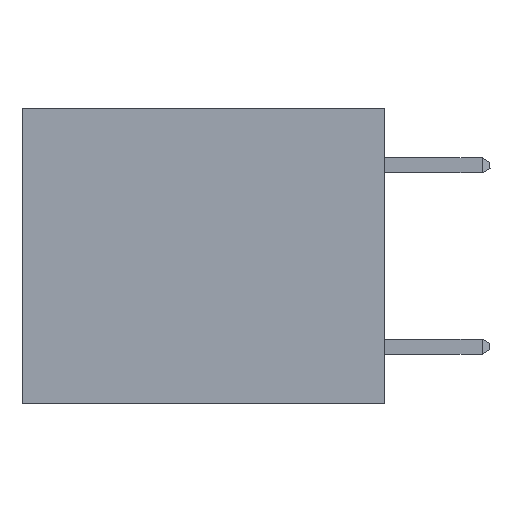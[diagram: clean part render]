
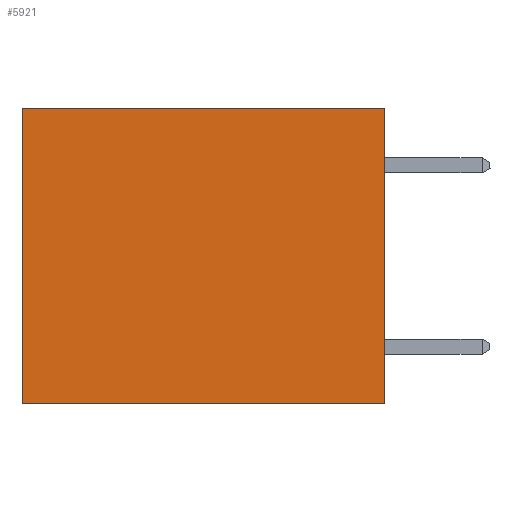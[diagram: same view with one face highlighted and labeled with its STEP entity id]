
A CAD part, left-side view. The second image highlights one B-rep face of the part: STEP entity #5921.
In plain terms, the highlighted planar face has unit normal (-1, 0, 0).
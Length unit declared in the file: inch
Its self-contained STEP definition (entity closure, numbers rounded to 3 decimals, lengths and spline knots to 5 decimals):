
#1148 = PLANE ( 'NONE',  #30560 ) ;
#2195 = ORIENTED_EDGE ( 'NONE', *, *, #9939, .F. ) ;
#3368 = CARTESIAN_POINT ( 'NONE',  ( 0.3165, 0., -0.49 ) ) ;
#4764 = DIRECTION ( 'NONE',  ( 0., 0., -1. ) ) ;
#5921 = ADVANCED_FACE ( 'NONE', ( #30733 ), #1148, .F. ) ;
#6543 = LINE ( 'NONE', #24455, #24176 ) ;
#6935 = VECTOR ( 'NONE', #18774, 39.37008 ) ;
#8947 = CARTESIAN_POINT ( 'NONE',  ( 0.3165, 0., -0.49 ) ) ;
#9203 = CARTESIAN_POINT ( 'NONE',  ( 0.3165, 0., 0. ) ) ;
#9793 = LINE ( 'NONE', #22160, #30605 ) ;
#9939 = EDGE_CURVE ( 'NONE', #31542, #16317, #9793, .T. ) ;
#10577 = ORIENTED_EDGE ( 'NONE', *, *, #11496, .F. ) ;
#10860 = VERTEX_POINT ( 'NONE', #31512 ) ;
#11496 = EDGE_CURVE ( 'NONE', #16317, #10860, #31246, .T. ) ;
#12301 = VECTOR ( 'NONE', #15707, 39.37008 ) ;
#12535 = EDGE_LOOP ( 'NONE', ( #29136, #10577, #2195, #23828 ) ) ;
#15707 = DIRECTION ( 'NONE',  ( 0., 1., 0. ) ) ;
#16317 = VERTEX_POINT ( 'NONE', #8947 ) ;
#17160 = EDGE_CURVE ( 'NONE', #18305, #10860, #6543, .T. ) ;
#18305 = VERTEX_POINT ( 'NONE', #22485 ) ;
#18774 = DIRECTION ( 'NONE',  ( 0., 1., 0. ) ) ;
#20648 = CARTESIAN_POINT ( 'NONE',  ( 0.3165, 0., 0. ) ) ;
#20927 = LINE ( 'NONE', #20648, #12301 ) ;
#20959 = CARTESIAN_POINT ( 'NONE',  ( 0.3165, 0., -0.49 ) ) ;
#22160 = CARTESIAN_POINT ( 'NONE',  ( 0.3165, 0., -0.49 ) ) ;
#22485 = CARTESIAN_POINT ( 'NONE',  ( 0.3165, 0.6, 0. ) ) ;
#23828 = ORIENTED_EDGE ( 'NONE', *, *, #31322, .T. ) ;
#24176 = VECTOR ( 'NONE', #29958, 39.37008 ) ;
#24455 = CARTESIAN_POINT ( 'NONE',  ( 0.3165, 0.6, -0.49 ) ) ;
#28544 = DIRECTION ( 'NONE',  ( 1., 0., 0. ) ) ;
#29136 = ORIENTED_EDGE ( 'NONE', *, *, #17160, .T. ) ;
#29958 = DIRECTION ( 'NONE',  ( 0., 0., -1. ) ) ;
#30560 = AXIS2_PLACEMENT_3D ( 'NONE', #20959, #28544, #31047 ) ;
#30605 = VECTOR ( 'NONE', #4764, 39.37008 ) ;
#30733 = FACE_OUTER_BOUND ( 'NONE', #12535, .T. ) ;
#31047 = DIRECTION ( 'NONE',  ( 0., 0., -1. ) ) ;
#31246 = LINE ( 'NONE', #3368, #6935 ) ;
#31322 = EDGE_CURVE ( 'NONE', #31542, #18305, #20927, .T. ) ;
#31512 = CARTESIAN_POINT ( 'NONE',  ( 0.3165, 0.6, -0.49 ) ) ;
#31542 = VERTEX_POINT ( 'NONE', #9203 ) ;
